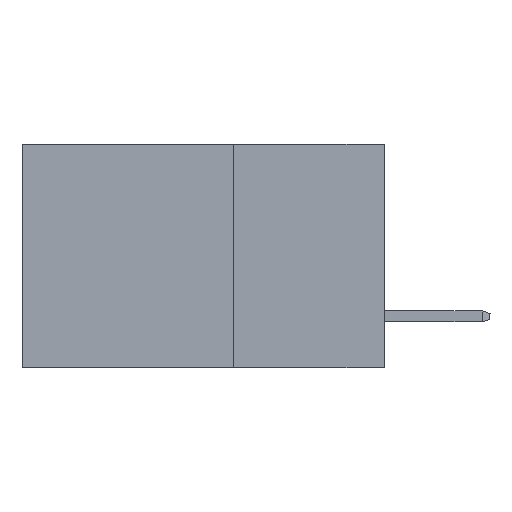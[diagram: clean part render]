
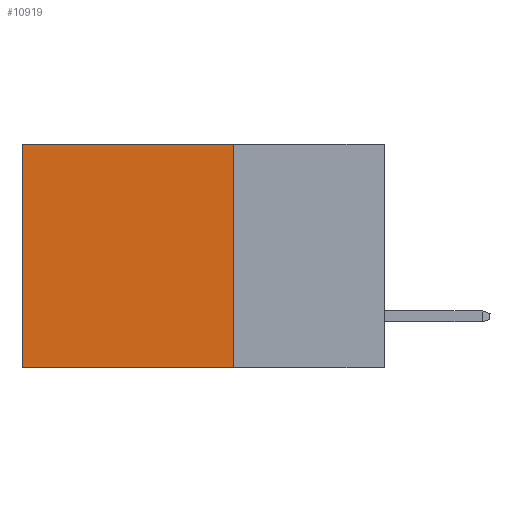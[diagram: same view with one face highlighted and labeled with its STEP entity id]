
A CAD part, left-side view. The second image highlights one B-rep face of the part: STEP entity #10919.
In plain terms, the highlighted planar face has unit normal (-1, 0, 0).
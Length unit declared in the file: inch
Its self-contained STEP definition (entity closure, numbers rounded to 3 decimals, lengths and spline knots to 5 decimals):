
#440 = LINE ( 'NONE', #14084, #11694 ) ;
#1471 = DIRECTION ( 'NONE',  ( 0., 1., 0. ) ) ;
#1521 = VECTOR ( 'NONE', #15374, 39.37008 ) ;
#1769 = VERTEX_POINT ( 'NONE', #5575 ) ;
#3558 = CARTESIAN_POINT ( 'NONE',  ( 0.2615, 0.6, -0.37 ) ) ;
#3641 = VERTEX_POINT ( 'NONE', #3558 ) ;
#3784 = DIRECTION ( 'NONE',  ( 0., 0., -1. ) ) ;
#4482 = DIRECTION ( 'NONE',  ( 1., 0., 0. ) ) ;
#5026 = LINE ( 'NONE', #15188, #7892 ) ;
#5575 = CARTESIAN_POINT ( 'NONE',  ( 0.2615, 0.6, 0. ) ) ;
#5707 = FACE_OUTER_BOUND ( 'NONE', #8621, .T. ) ;
#5785 = ORIENTED_EDGE ( 'NONE', *, *, #9901, .F. ) ;
#6026 = ORIENTED_EDGE ( 'NONE', *, *, #14691, .F. ) ;
#6283 = LINE ( 'NONE', #12719, #1521 ) ;
#7275 = EDGE_CURVE ( 'NONE', #14077, #1769, #11464, .T. ) ;
#7741 = CARTESIAN_POINT ( 'NONE',  ( 0.2615, 0.25, 0. ) ) ;
#7885 = DIRECTION ( 'NONE',  ( 0., 0., -1. ) ) ;
#7892 = VECTOR ( 'NONE', #3784, 39.37008 ) ;
#8621 = EDGE_LOOP ( 'NONE', ( #16337, #5785, #6026, #11407 ) ) ;
#9578 = DIRECTION ( 'NONE',  ( 0., 0., -1. ) ) ;
#9705 = AXIS2_PLACEMENT_3D ( 'NONE', #11911, #4482, #9578 ) ;
#9901 = EDGE_CURVE ( 'NONE', #12612, #3641, #6283, .T. ) ;
#10655 = CARTESIAN_POINT ( 'NONE',  ( 0.2615, 0.25, 0. ) ) ;
#10755 = PLANE ( 'NONE',  #9705 ) ;
#10919 = ADVANCED_FACE ( 'NONE', ( #5707 ), #10755, .F. ) ;
#11407 = ORIENTED_EDGE ( 'NONE', *, *, #7275, .T. ) ;
#11464 = LINE ( 'NONE', #7741, #15703 ) ;
#11566 = EDGE_CURVE ( 'NONE', #1769, #3641, #5026, .T. ) ;
#11694 = VECTOR ( 'NONE', #7885, 39.37008 ) ;
#11911 = CARTESIAN_POINT ( 'NONE',  ( 0.2615, 0.25, -0.37 ) ) ;
#12612 = VERTEX_POINT ( 'NONE', #14284 ) ;
#12719 = CARTESIAN_POINT ( 'NONE',  ( 0.2615, 0.25, -0.37 ) ) ;
#14077 = VERTEX_POINT ( 'NONE', #10655 ) ;
#14084 = CARTESIAN_POINT ( 'NONE',  ( 0.2615, 0.25, -0.37 ) ) ;
#14284 = CARTESIAN_POINT ( 'NONE',  ( 0.2615, 0.25, -0.37 ) ) ;
#14691 = EDGE_CURVE ( 'NONE', #14077, #12612, #440, .T. ) ;
#15188 = CARTESIAN_POINT ( 'NONE',  ( 0.2615, 0.6, -0.37 ) ) ;
#15374 = DIRECTION ( 'NONE',  ( 0., 1., 0. ) ) ;
#15703 = VECTOR ( 'NONE', #1471, 39.37008 ) ;
#16337 = ORIENTED_EDGE ( 'NONE', *, *, #11566, .T. ) ;
